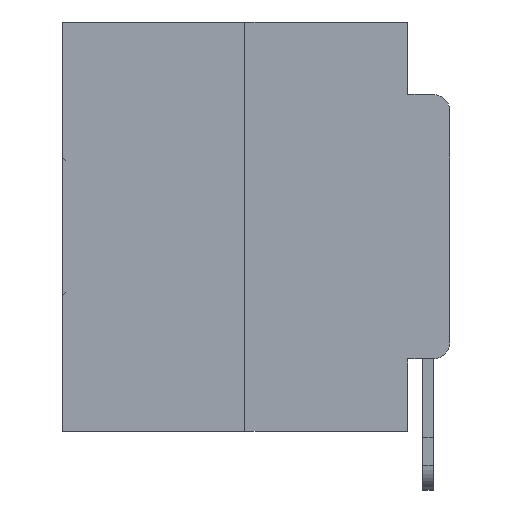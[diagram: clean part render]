
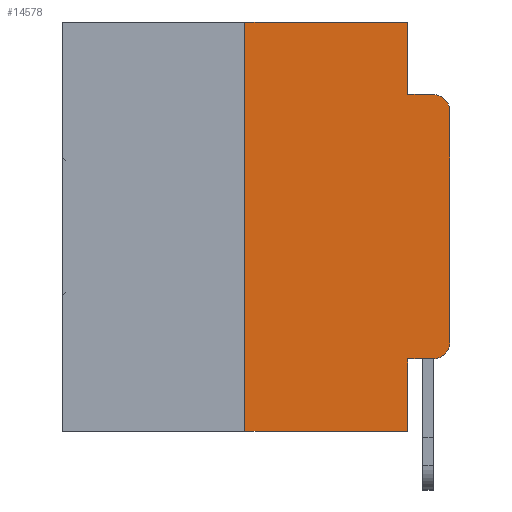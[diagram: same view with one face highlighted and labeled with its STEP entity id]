
A CAD part, left-side view. The second image highlights one B-rep face of the part: STEP entity #14578.
In plain terms, the highlighted planar face has unit normal (-1, 0, 0).
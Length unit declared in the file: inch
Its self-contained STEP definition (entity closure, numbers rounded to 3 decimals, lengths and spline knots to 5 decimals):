
#39 = ORIENTED_EDGE ( 'NONE', *, *, #22583, .F. ) ;
#964 = LINE ( 'NONE', #4329, #26102 ) ;
#1240 = VECTOR ( 'NONE', #4688, 39.37008 ) ;
#1591 = LINE ( 'NONE', #23897, #14263 ) ;
#1655 = VERTEX_POINT ( 'NONE', #28968 ) ;
#1738 = CARTESIAN_POINT ( 'NONE',  ( 0., 0.25, 0. ) ) ;
#1988 = CARTESIAN_POINT ( 'NONE',  ( 0., 0.051, 0. ) ) ;
#2398 = EDGE_CURVE ( 'NONE', #12861, #6796, #25596, .T. ) ;
#4329 = CARTESIAN_POINT ( 'NONE',  ( 0., 0.051, -0.0885 ) ) ;
#4645 = EDGE_CURVE ( 'NONE', #26656, #29672, #13369, .T. ) ;
#4688 = DIRECTION ( 'NONE',  ( 0., 0., -1. ) ) ;
#4847 = FACE_OUTER_BOUND ( 'NONE', #31192, .T. ) ;
#4851 = EDGE_CURVE ( 'NONE', #9191, #12593, #12975, .T. ) ;
#5404 = AXIS2_PLACEMENT_3D ( 'NONE', #7645, #10191, #26532 ) ;
#5496 = ORIENTED_EDGE ( 'NONE', *, *, #28841, .T. ) ;
#6643 = VECTOR ( 'NONE', #27716, 39.37008 ) ;
#6796 = VERTEX_POINT ( 'NONE', #1738 ) ;
#6841 = CARTESIAN_POINT ( 'NONE',  ( 0., 0., -0.1085 ) ) ;
#7645 = CARTESIAN_POINT ( 'NONE',  ( 0., 0.473, 0. ) ) ;
#7782 = CARTESIAN_POINT ( 'NONE',  ( 0., 0.473, -0.5 ) ) ;
#8126 = EDGE_CURVE ( 'NONE', #29729, #26656, #22771, .T. ) ;
#9191 = VERTEX_POINT ( 'NONE', #9716 ) ;
#9441 = CARTESIAN_POINT ( 'NONE',  ( 0., 0.02, -0.1085 ) ) ;
#9716 = CARTESIAN_POINT ( 'NONE',  ( 0., 0.051, -0.4115 ) ) ;
#9744 = VECTOR ( 'NONE', #10327, 39.37008 ) ;
#9912 = CARTESIAN_POINT ( 'NONE',  ( 0., 0.02, -0.0885 ) ) ;
#10191 = DIRECTION ( 'NONE',  ( 1., 0., 0. ) ) ;
#10325 = VECTOR ( 'NONE', #25383, 39.37008 ) ;
#10327 = DIRECTION ( 'NONE',  ( 0., -1., 0. ) ) ;
#10679 = ORIENTED_EDGE ( 'NONE', *, *, #2398, .F. ) ;
#10755 = CARTESIAN_POINT ( 'NONE',  ( 0., 0.02, -0.4115 ) ) ;
#11040 = EDGE_CURVE ( 'NONE', #17971, #26074, #15425, .T. ) ;
#11061 = ORIENTED_EDGE ( 'NONE', *, *, #16957, .T. ) ;
#11883 = DIRECTION ( 'NONE',  ( 0., 0., -1. ) ) ;
#12593 = VERTEX_POINT ( 'NONE', #10755 ) ;
#12861 = VERTEX_POINT ( 'NONE', #13951 ) ;
#12975 = LINE ( 'NONE', #24432, #30801 ) ;
#13369 = CIRCLE ( 'NONE', #25793, 0.02 ) ;
#13804 = CARTESIAN_POINT ( 'NONE',  ( 0., 0.02, -0.3915 ) ) ;
#13951 = CARTESIAN_POINT ( 'NONE',  ( 0., 0.25, -0.5 ) ) ;
#14263 = VECTOR ( 'NONE', #26239, 39.37008 ) ;
#14578 = ADVANCED_FACE ( 'NONE', ( #4847 ), #21877, .F. ) ;
#15425 = LINE ( 'NONE', #1988, #1240 ) ;
#16168 = DIRECTION ( 'NONE',  ( 0., 0., -1. ) ) ;
#16460 = EDGE_CURVE ( 'NONE', #6796, #17971, #28236, .T. ) ;
#16574 = ORIENTED_EDGE ( 'NONE', *, *, #4645, .T. ) ;
#16957 = EDGE_CURVE ( 'NONE', #12593, #29729, #18314, .T. ) ;
#17971 = VERTEX_POINT ( 'NONE', #24032 ) ;
#18314 = CIRCLE ( 'NONE', #24281, 0.02 ) ;
#19521 = CARTESIAN_POINT ( 'NONE',  ( 0., 0.473, 0. ) ) ;
#21174 = CARTESIAN_POINT ( 'NONE',  ( 0., 0.051, -0.0885 ) ) ;
#21295 = ORIENTED_EDGE ( 'NONE', *, *, #8126, .T. ) ;
#21358 = VECTOR ( 'NONE', #21830, 39.37008 ) ;
#21830 = DIRECTION ( 'NONE',  ( 0., -1., 0. ) ) ;
#21877 = PLANE ( 'NONE',  #5404 ) ;
#22043 = ORIENTED_EDGE ( 'NONE', *, *, #4851, .T. ) ;
#22583 = EDGE_CURVE ( 'NONE', #9191, #1655, #1591, .T. ) ;
#22771 = LINE ( 'NONE', #23043, #10325 ) ;
#23043 = CARTESIAN_POINT ( 'NONE',  ( 0., 0., 0. ) ) ;
#23897 = CARTESIAN_POINT ( 'NONE',  ( 0., 0.051, 0. ) ) ;
#24032 = CARTESIAN_POINT ( 'NONE',  ( 0., 0.051, 0. ) ) ;
#24281 = AXIS2_PLACEMENT_3D ( 'NONE', #13804, #30048, #16168 ) ;
#24432 = CARTESIAN_POINT ( 'NONE',  ( 0., 0.051, -0.4115 ) ) ;
#24911 = ORIENTED_EDGE ( 'NONE', *, *, #26110, .F. ) ;
#25379 = CARTESIAN_POINT ( 'NONE',  ( 0., 0.25, 0. ) ) ;
#25383 = DIRECTION ( 'NONE',  ( 0., 0., 1. ) ) ;
#25596 = LINE ( 'NONE', #25379, #6643 ) ;
#25793 = AXIS2_PLACEMENT_3D ( 'NONE', #9441, #25873, #11883 ) ;
#25873 = DIRECTION ( 'NONE',  ( -1., 0., 0. ) ) ;
#26074 = VERTEX_POINT ( 'NONE', #21174 ) ;
#26102 = VECTOR ( 'NONE', #28248, 39.37008 ) ;
#26110 = EDGE_CURVE ( 'NONE', #26074, #29672, #964, .T. ) ;
#26239 = DIRECTION ( 'NONE',  ( 0., 0., -1. ) ) ;
#26532 = DIRECTION ( 'NONE',  ( 0., 0., -1. ) ) ;
#26656 = VERTEX_POINT ( 'NONE', #6841 ) ;
#27100 = ORIENTED_EDGE ( 'NONE', *, *, #11040, .F. ) ;
#27716 = DIRECTION ( 'NONE',  ( 0., 0., 1. ) ) ;
#28236 = LINE ( 'NONE', #19521, #21358 ) ;
#28248 = DIRECTION ( 'NONE',  ( 0., -1., 0. ) ) ;
#28538 = ORIENTED_EDGE ( 'NONE', *, *, #16460, .F. ) ;
#28841 = EDGE_CURVE ( 'NONE', #12861, #1655, #29139, .T. ) ;
#28968 = CARTESIAN_POINT ( 'NONE',  ( 0., 0.051, -0.5 ) ) ;
#29086 = DIRECTION ( 'NONE',  ( 0., -1., 0. ) ) ;
#29139 = LINE ( 'NONE', #7782, #9744 ) ;
#29672 = VERTEX_POINT ( 'NONE', #9912 ) ;
#29729 = VERTEX_POINT ( 'NONE', #31039 ) ;
#30048 = DIRECTION ( 'NONE',  ( -1., 0., 0. ) ) ;
#30801 = VECTOR ( 'NONE', #29086, 39.37008 ) ;
#31039 = CARTESIAN_POINT ( 'NONE',  ( 0., 0., -0.3915 ) ) ;
#31192 = EDGE_LOOP ( 'NONE', ( #21295, #16574, #24911, #27100, #28538, #10679, #5496, #39, #22043, #11061 ) ) ;
